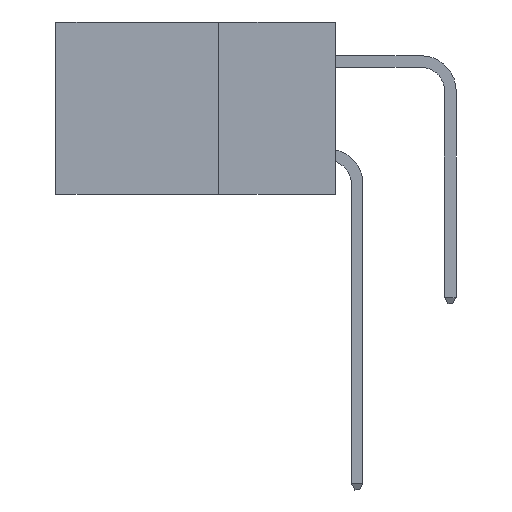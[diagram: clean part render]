
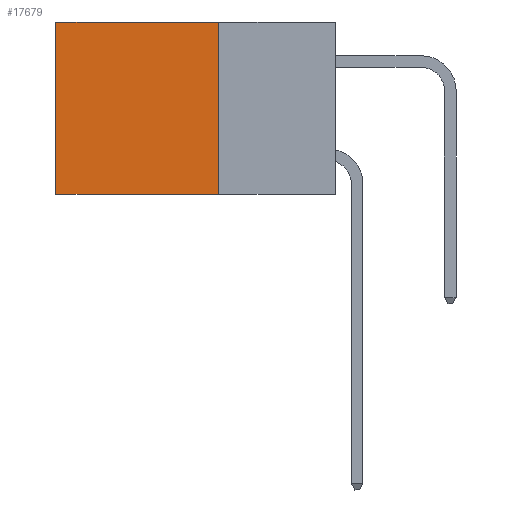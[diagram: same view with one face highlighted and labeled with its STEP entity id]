
A CAD part, left-side view. The second image highlights one B-rep face of the part: STEP entity #17679.
In plain terms, the highlighted planar face has unit normal (-1, 0, 0).
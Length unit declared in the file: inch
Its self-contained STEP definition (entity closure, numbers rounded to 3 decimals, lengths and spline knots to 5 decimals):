
#582 = FACE_OUTER_BOUND ( 'NONE', #3465, .T. ) ;
#589 = LINE ( 'NONE', #15398, #2426 ) ;
#785 = CARTESIAN_POINT ( 'NONE',  ( 0.2875, 0.6, 0. ) ) ;
#1885 = DIRECTION ( 'NONE',  ( 0., 0., -1. ) ) ;
#2426 = VECTOR ( 'NONE', #22795, 39.37008 ) ;
#3157 = DIRECTION ( 'NONE',  ( 1., 0., 0. ) ) ;
#3465 = EDGE_LOOP ( 'NONE', ( #30237, #25512, #13322, #6094 ) ) ;
#3762 = LINE ( 'NONE', #13413, #27632 ) ;
#4294 = LINE ( 'NONE', #23931, #15496 ) ;
#6094 = ORIENTED_EDGE ( 'NONE', *, *, #9754, .T. ) ;
#6790 = LINE ( 'NONE', #28547, #19213 ) ;
#7214 = CARTESIAN_POINT ( 'NONE',  ( 0.2875, 0.25, -0.37 ) ) ;
#7814 = PLANE ( 'NONE',  #10538 ) ;
#9754 = EDGE_CURVE ( 'NONE', #11775, #22866, #6790, .T. ) ;
#9852 = VERTEX_POINT ( 'NONE', #13754 ) ;
#10346 = DIRECTION ( 'NONE',  ( 0., 0., -1. ) ) ;
#10398 = EDGE_CURVE ( 'NONE', #25355, #9852, #589, .T. ) ;
#10538 = AXIS2_PLACEMENT_3D ( 'NONE', #30370, #3157, #20219 ) ;
#11775 = VERTEX_POINT ( 'NONE', #18659 ) ;
#13322 = ORIENTED_EDGE ( 'NONE', *, *, #25736, .F. ) ;
#13413 = CARTESIAN_POINT ( 'NONE',  ( 0.2875, 0.6, 0. ) ) ;
#13754 = CARTESIAN_POINT ( 'NONE',  ( 0.2875, 0.6, -0.37 ) ) ;
#15398 = CARTESIAN_POINT ( 'NONE',  ( 0.2875, 0.25, -0.37 ) ) ;
#15496 = VECTOR ( 'NONE', #1885, 39.37008 ) ;
#16323 = DIRECTION ( 'NONE',  ( 0., 1., 0. ) ) ;
#17679 = ADVANCED_FACE ( 'NONE', ( #582 ), #7814, .F. ) ;
#18659 = CARTESIAN_POINT ( 'NONE',  ( 0.2875, 0.25, 0. ) ) ;
#19213 = VECTOR ( 'NONE', #16323, 39.37008 ) ;
#20219 = DIRECTION ( 'NONE',  ( 0., 0., -1. ) ) ;
#20650 = EDGE_CURVE ( 'NONE', #22866, #9852, #3762, .T. ) ;
#22795 = DIRECTION ( 'NONE',  ( 0., 1., 0. ) ) ;
#22866 = VERTEX_POINT ( 'NONE', #785 ) ;
#23931 = CARTESIAN_POINT ( 'NONE',  ( 0.2875, 0.25, 0. ) ) ;
#25355 = VERTEX_POINT ( 'NONE', #7214 ) ;
#25512 = ORIENTED_EDGE ( 'NONE', *, *, #10398, .F. ) ;
#25736 = EDGE_CURVE ( 'NONE', #11775, #25355, #4294, .T. ) ;
#27632 = VECTOR ( 'NONE', #10346, 39.37008 ) ;
#28547 = CARTESIAN_POINT ( 'NONE',  ( 0.2875, 0.25, 0. ) ) ;
#30237 = ORIENTED_EDGE ( 'NONE', *, *, #20650, .T. ) ;
#30370 = CARTESIAN_POINT ( 'NONE',  ( 0.2875, 0.25, 0. ) ) ;
